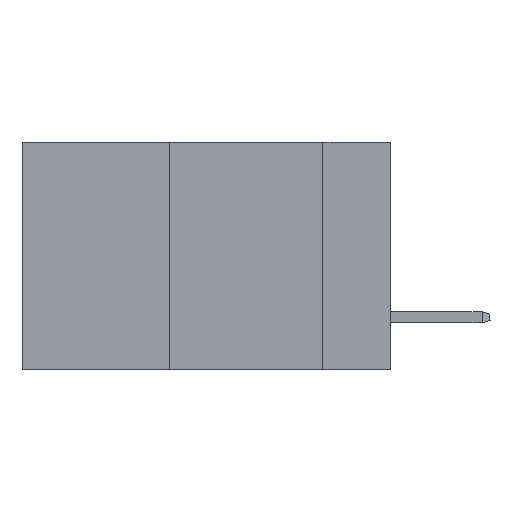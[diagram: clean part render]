
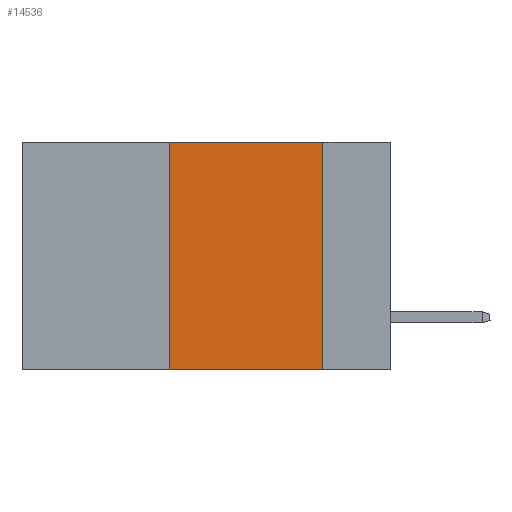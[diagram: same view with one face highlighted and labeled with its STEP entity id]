
A CAD part, left-side view. The second image highlights one B-rep face of the part: STEP entity #14536.
In plain terms, the highlighted planar face has unit normal (-1, 0, 0).
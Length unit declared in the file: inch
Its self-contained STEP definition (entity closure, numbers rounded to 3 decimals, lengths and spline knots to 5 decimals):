
#1768 = LINE ( 'NONE', #29443, #11935 ) ;
#7146 = LINE ( 'NONE', #28676, #11180 ) ;
#7805 = VECTOR ( 'NONE', #20660, 39.37008 ) ;
#7843 = ORIENTED_EDGE ( 'NONE', *, *, #19829, .F. ) ;
#8414 = CARTESIAN_POINT ( 'NONE',  ( 0., 0.6, -0.37 ) ) ;
#8836 = ORIENTED_EDGE ( 'NONE', *, *, #32066, .F. ) ;
#9112 = VERTEX_POINT ( 'NONE', #15136 ) ;
#9531 = VECTOR ( 'NONE', #34186, 39.37008 ) ;
#9708 = DIRECTION ( 'NONE',  ( 0., 0., -1. ) ) ;
#10962 = VERTEX_POINT ( 'NONE', #29017 ) ;
#11180 = VECTOR ( 'NONE', #32164, 39.37008 ) ;
#11882 = CARTESIAN_POINT ( 'NONE',  ( 0., 0.11, -0.37 ) ) ;
#11935 = VECTOR ( 'NONE', #9708, 39.37008 ) ;
#12882 = PLANE ( 'NONE',  #27296 ) ;
#13025 = DIRECTION ( 'NONE',  ( 0., 0., -1. ) ) ;
#13820 = ORIENTED_EDGE ( 'NONE', *, *, #28006, .F. ) ;
#14206 = VERTEX_POINT ( 'NONE', #11882 ) ;
#14536 = ADVANCED_FACE ( 'NONE', ( #21152 ), #12882, .F. ) ;
#15136 = CARTESIAN_POINT ( 'NONE',  ( 0., 0.36, -0.37 ) ) ;
#15744 = DIRECTION ( 'NONE',  ( 1., 0., 0. ) ) ;
#17130 = LINE ( 'NONE', #32099, #7805 ) ;
#19829 = EDGE_CURVE ( 'NONE', #10962, #14206, #1768, .T. ) ;
#20083 = EDGE_LOOP ( 'NONE', ( #7843, #13820, #8836, #36747 ) ) ;
#20660 = DIRECTION ( 'NONE',  ( 0., 0., 1. ) ) ;
#21152 = FACE_OUTER_BOUND ( 'NONE', #20083, .T. ) ;
#22467 = LINE ( 'NONE', #8414, #9531 ) ;
#27296 = AXIS2_PLACEMENT_3D ( 'NONE', #32713, #15744, #13025 ) ;
#27496 = CARTESIAN_POINT ( 'NONE',  ( 0., 0.36, 0. ) ) ;
#28006 = EDGE_CURVE ( 'NONE', #31599, #10962, #7146, .T. ) ;
#28676 = CARTESIAN_POINT ( 'NONE',  ( 0., 0.6, 0. ) ) ;
#29017 = CARTESIAN_POINT ( 'NONE',  ( 0., 0.11, 0. ) ) ;
#29443 = CARTESIAN_POINT ( 'NONE',  ( 0., 0.11, 0. ) ) ;
#31599 = VERTEX_POINT ( 'NONE', #27496 ) ;
#32066 = EDGE_CURVE ( 'NONE', #9112, #31599, #17130, .T. ) ;
#32099 = CARTESIAN_POINT ( 'NONE',  ( 0., 0.36, 0. ) ) ;
#32164 = DIRECTION ( 'NONE',  ( 0., -1., 0. ) ) ;
#32713 = CARTESIAN_POINT ( 'NONE',  ( 0., 0.6, 0. ) ) ;
#32981 = EDGE_CURVE ( 'NONE', #9112, #14206, #22467, .T. ) ;
#34186 = DIRECTION ( 'NONE',  ( 0., -1., 0. ) ) ;
#36747 = ORIENTED_EDGE ( 'NONE', *, *, #32981, .T. ) ;
